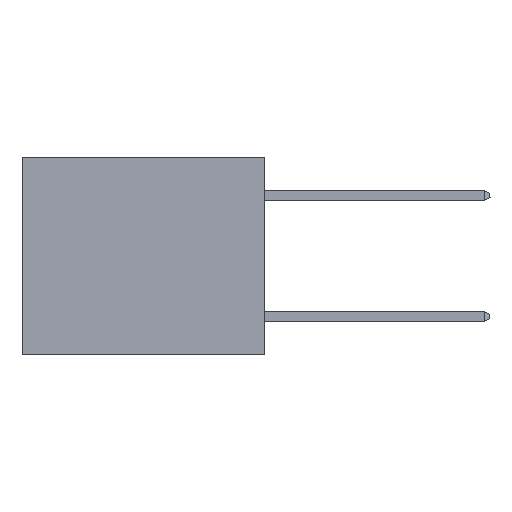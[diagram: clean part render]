
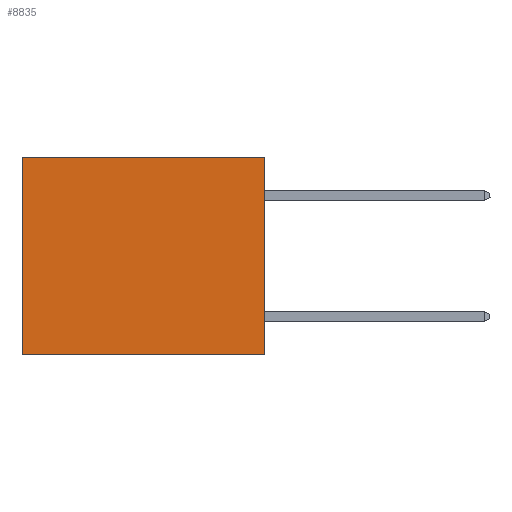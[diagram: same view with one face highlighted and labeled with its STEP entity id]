
A CAD part, left-side view. The second image highlights one B-rep face of the part: STEP entity #8835.
In plain terms, the highlighted planar face has unit normal (-1, 0, 0).
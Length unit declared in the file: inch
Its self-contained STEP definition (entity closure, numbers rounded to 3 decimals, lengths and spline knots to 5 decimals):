
#278 = VERTEX_POINT ( 'NONE', #24867 ) ;
#806 = CARTESIAN_POINT ( 'NONE',  ( 0.3165, 0.6, -0.49 ) ) ;
#1124 = VERTEX_POINT ( 'NONE', #23611 ) ;
#1281 = CARTESIAN_POINT ( 'NONE',  ( 0.3165, 0., -0.49 ) ) ;
#1469 = CARTESIAN_POINT ( 'NONE',  ( 0.3165, 0., -0.49 ) ) ;
#2426 = ORIENTED_EDGE ( 'NONE', *, *, #7517, .T. ) ;
#2784 = CARTESIAN_POINT ( 'NONE',  ( 0.3165, 0.6, 0. ) ) ;
#5762 = AXIS2_PLACEMENT_3D ( 'NONE', #6134, #13345, #23844 ) ;
#6134 = CARTESIAN_POINT ( 'NONE',  ( 0.3165, 0., -0.49 ) ) ;
#6148 = EDGE_LOOP ( 'NONE', ( #18386, #16146, #15072, #2426 ) ) ;
#6531 = VECTOR ( 'NONE', #19013, 39.37008 ) ;
#7517 = EDGE_CURVE ( 'NONE', #1124, #19967, #23855, .T. ) ;
#8835 = ADVANCED_FACE ( 'NONE', ( #13828 ), #18631, .F. ) ;
#9643 = VECTOR ( 'NONE', #27004, 39.37008 ) ;
#10188 = CARTESIAN_POINT ( 'NONE',  ( 0.3165, 0., 0. ) ) ;
#10408 = LINE ( 'NONE', #806, #11594 ) ;
#10423 = LINE ( 'NONE', #1469, #9643 ) ;
#11594 = VECTOR ( 'NONE', #29007, 39.37008 ) ;
#13345 = DIRECTION ( 'NONE',  ( 1., 0., 0. ) ) ;
#13828 = FACE_OUTER_BOUND ( 'NONE', #6148, .T. ) ;
#15072 = ORIENTED_EDGE ( 'NONE', *, *, #21261, .F. ) ;
#15883 = VECTOR ( 'NONE', #22651, 39.37008 ) ;
#16146 = ORIENTED_EDGE ( 'NONE', *, *, #21612, .F. ) ;
#18386 = ORIENTED_EDGE ( 'NONE', *, *, #24510, .T. ) ;
#18631 = PLANE ( 'NONE',  #5762 ) ;
#19013 = DIRECTION ( 'NONE',  ( 0., 0., -1. ) ) ;
#19967 = VERTEX_POINT ( 'NONE', #2784 ) ;
#21261 = EDGE_CURVE ( 'NONE', #1124, #27277, #25189, .T. ) ;
#21612 = EDGE_CURVE ( 'NONE', #27277, #278, #10423, .T. ) ;
#22651 = DIRECTION ( 'NONE',  ( 0., 1., 0. ) ) ;
#23611 = CARTESIAN_POINT ( 'NONE',  ( 0.3165, 0., 0. ) ) ;
#23844 = DIRECTION ( 'NONE',  ( 0., 0., -1. ) ) ;
#23855 = LINE ( 'NONE', #10188, #15883 ) ;
#24510 = EDGE_CURVE ( 'NONE', #19967, #278, #10408, .T. ) ;
#24867 = CARTESIAN_POINT ( 'NONE',  ( 0.3165, 0.6, -0.49 ) ) ;
#25189 = LINE ( 'NONE', #1281, #6531 ) ;
#26752 = CARTESIAN_POINT ( 'NONE',  ( 0.3165, 0., -0.49 ) ) ;
#27004 = DIRECTION ( 'NONE',  ( 0., 1., 0. ) ) ;
#27277 = VERTEX_POINT ( 'NONE', #26752 ) ;
#29007 = DIRECTION ( 'NONE',  ( 0., 0., -1. ) ) ;
